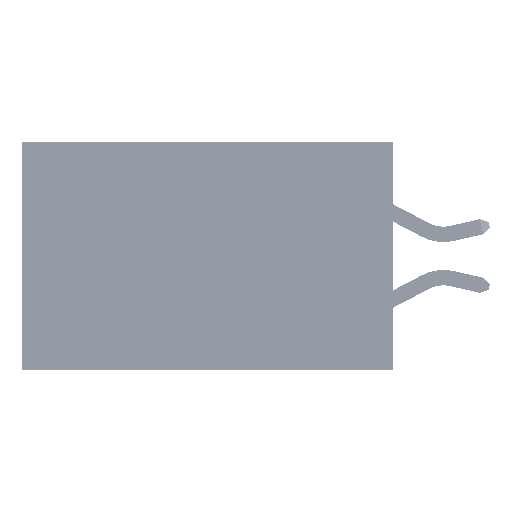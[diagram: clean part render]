
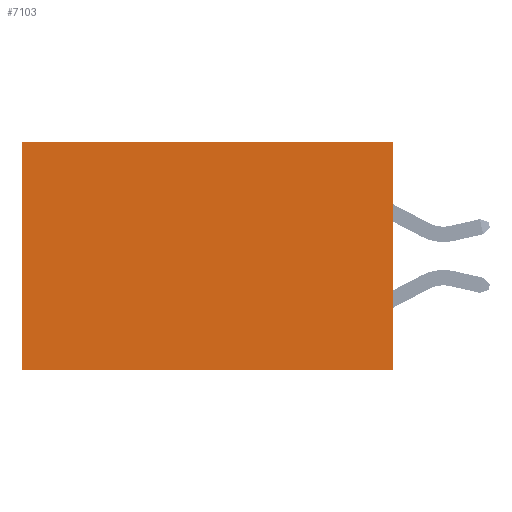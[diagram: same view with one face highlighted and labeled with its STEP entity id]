
A CAD part, left-side view. The second image highlights one B-rep face of the part: STEP entity #7103.
In plain terms, the highlighted planar face has unit normal (-1, 0, 0).
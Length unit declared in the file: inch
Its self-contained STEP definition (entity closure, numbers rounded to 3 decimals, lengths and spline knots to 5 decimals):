
#1513 = VERTEX_POINT ( 'NONE', #23924 ) ;
#1640 = VECTOR ( 'NONE', #47863, 39.37008 ) ;
#4395 = LINE ( 'NONE', #31858, #20487 ) ;
#6802 = DIRECTION ( 'NONE',  ( 0., 1., 0. ) ) ;
#7103 = ADVANCED_FACE ( 'NONE', ( #12717 ), #43357, .F. ) ;
#7191 = VERTEX_POINT ( 'NONE', #48664 ) ;
#7960 = DIRECTION ( 'NONE',  ( 0., 0., -1. ) ) ;
#8613 = EDGE_CURVE ( 'NONE', #23871, #7191, #4395, .T. ) ;
#10944 = CARTESIAN_POINT ( 'NONE',  ( 0.2875, 0., 0. ) ) ;
#12090 = CARTESIAN_POINT ( 'NONE',  ( 0.2875, 0., 0. ) ) ;
#12143 = DIRECTION ( 'NONE',  ( 0., 0., -1. ) ) ;
#12717 = FACE_OUTER_BOUND ( 'NONE', #26992, .T. ) ;
#16513 = ORIENTED_EDGE ( 'NONE', *, *, #22910, .F. ) ;
#16596 = VECTOR ( 'NONE', #50448, 39.37008 ) ;
#20487 = VECTOR ( 'NONE', #12143, 39.37008 ) ;
#22910 = EDGE_CURVE ( 'NONE', #26552, #1513, #30789, .T. ) ;
#23871 = VERTEX_POINT ( 'NONE', #45384 ) ;
#23924 = CARTESIAN_POINT ( 'NONE',  ( 0.2875, 0., -0.37 ) ) ;
#26552 = VERTEX_POINT ( 'NONE', #49313 ) ;
#26992 = EDGE_LOOP ( 'NONE', ( #37494, #51051, #16513, #49977 ) ) ;
#27137 = VECTOR ( 'NONE', #6802, 39.37008 ) ;
#29288 = AXIS2_PLACEMENT_3D ( 'NONE', #12090, #43858, #7960 ) ;
#30102 = LINE ( 'NONE', #48199, #1640 ) ;
#30789 = LINE ( 'NONE', #10944, #16596 ) ;
#31858 = CARTESIAN_POINT ( 'NONE',  ( 0.2875, 0.6, 0. ) ) ;
#37494 = ORIENTED_EDGE ( 'NONE', *, *, #8613, .T. ) ;
#37821 = EDGE_CURVE ( 'NONE', #1513, #7191, #30102, .T. ) ;
#38316 = LINE ( 'NONE', #38407, #27137 ) ;
#38407 = CARTESIAN_POINT ( 'NONE',  ( 0.2875, 0., 0. ) ) ;
#43357 = PLANE ( 'NONE',  #29288 ) ;
#43858 = DIRECTION ( 'NONE',  ( 1., 0., 0. ) ) ;
#45384 = CARTESIAN_POINT ( 'NONE',  ( 0.2875, 0.6, 0. ) ) ;
#47073 = EDGE_CURVE ( 'NONE', #26552, #23871, #38316, .T. ) ;
#47863 = DIRECTION ( 'NONE',  ( 0., 1., 0. ) ) ;
#48199 = CARTESIAN_POINT ( 'NONE',  ( 0.2875, 0., -0.37 ) ) ;
#48664 = CARTESIAN_POINT ( 'NONE',  ( 0.2875, 0.6, -0.37 ) ) ;
#49313 = CARTESIAN_POINT ( 'NONE',  ( 0.2875, 0., 0. ) ) ;
#49977 = ORIENTED_EDGE ( 'NONE', *, *, #47073, .T. ) ;
#50448 = DIRECTION ( 'NONE',  ( 0., 0., -1. ) ) ;
#51051 = ORIENTED_EDGE ( 'NONE', *, *, #37821, .F. ) ;
